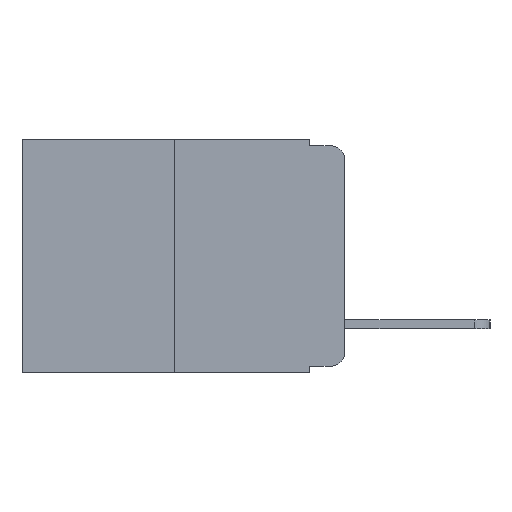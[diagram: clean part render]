
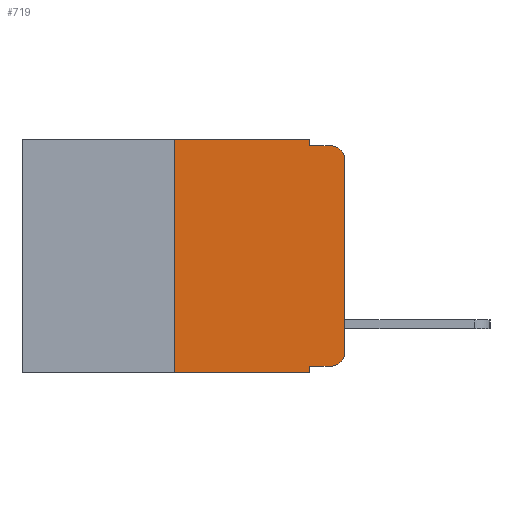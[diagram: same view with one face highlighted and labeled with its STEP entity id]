
A CAD part, left-side view. The second image highlights one B-rep face of the part: STEP entity #719.
In plain terms, the highlighted planar face has unit normal (-1, 0, 0).
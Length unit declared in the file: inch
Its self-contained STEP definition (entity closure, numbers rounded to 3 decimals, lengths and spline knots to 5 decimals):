
#85 = DIRECTION ( 'NONE',  ( 0., 0., 1. ) ) ;
#147 = ORIENTED_EDGE ( 'NONE', *, *, #9426, .F. ) ;
#243 = AXIS2_PLACEMENT_3D ( 'NONE', #4914, #6221, #6185 ) ;
#519 = FACE_OUTER_BOUND ( 'NONE', #11631, .T. ) ;
#551 = EDGE_CURVE ( 'NONE', #7338, #7774, #8680, .T. ) ;
#719 = ADVANCED_FACE ( 'NONE', ( #519 ), #4931, .F. ) ;
#1173 = DIRECTION ( 'NONE',  ( 0., -1., 0. ) ) ;
#1215 = ORIENTED_EDGE ( 'NONE', *, *, #3487, .T. ) ;
#1494 = CARTESIAN_POINT ( 'NONE',  ( 0., 0.02, -0.333 ) ) ;
#1681 = EDGE_CURVE ( 'NONE', #10068, #3542, #5130, .T. ) ;
#1827 = CARTESIAN_POINT ( 'NONE',  ( 0., 0.25, 0. ) ) ;
#1839 = CARTESIAN_POINT ( 'NONE',  ( 0., 0.02, -0.313 ) ) ;
#1917 = VECTOR ( 'NONE', #4175, 39.37008 ) ;
#1948 = CARTESIAN_POINT ( 'NONE',  ( 0., 0.02, -0.03 ) ) ;
#1987 = CIRCLE ( 'NONE', #7078, 0.02 ) ;
#2053 = EDGE_CURVE ( 'NONE', #7774, #11723, #11647, .T. ) ;
#2371 = CARTESIAN_POINT ( 'NONE',  ( 0., 0., 0. ) ) ;
#2797 = VECTOR ( 'NONE', #3889, 39.37008 ) ;
#2840 = CIRCLE ( 'NONE', #4046, 0.02 ) ;
#2930 = DIRECTION ( 'NONE',  ( 0., 0., -1. ) ) ;
#2997 = DIRECTION ( 'NONE',  ( 0., -1., 0. ) ) ;
#3046 = DIRECTION ( 'NONE',  ( 0., 0., -1. ) ) ;
#3122 = ORIENTED_EDGE ( 'NONE', *, *, #8035, .T. ) ;
#3487 = EDGE_CURVE ( 'NONE', #10880, #11723, #2840, .T. ) ;
#3542 = VERTEX_POINT ( 'NONE', #11467 ) ;
#3755 = EDGE_CURVE ( 'NONE', #8293, #7015, #1987, .T. ) ;
#3889 = DIRECTION ( 'NONE',  ( 0., -1., 0. ) ) ;
#3896 = VERTEX_POINT ( 'NONE', #4187 ) ;
#4046 = AXIS2_PLACEMENT_3D ( 'NONE', #1948, #8791, #3046 ) ;
#4175 = DIRECTION ( 'NONE',  ( 0., 0., -1. ) ) ;
#4187 = CARTESIAN_POINT ( 'NONE',  ( 0., 0.25, 0. ) ) ;
#4394 = CARTESIAN_POINT ( 'NONE',  ( 0., 0.473, -0.343 ) ) ;
#4571 = CARTESIAN_POINT ( 'NONE',  ( 0., 0.051, 0. ) ) ;
#4580 = ORIENTED_EDGE ( 'NONE', *, *, #5745, .T. ) ;
#4914 = CARTESIAN_POINT ( 'NONE',  ( 0., 0.473, 0. ) ) ;
#4931 = PLANE ( 'NONE',  #243 ) ;
#5130 = LINE ( 'NONE', #4394, #11792 ) ;
#5489 = LINE ( 'NONE', #8634, #2797 ) ;
#5745 = EDGE_CURVE ( 'NONE', #9624, #8293, #5489, .T. ) ;
#6185 = DIRECTION ( 'NONE',  ( 0., 0., -1. ) ) ;
#6221 = DIRECTION ( 'NONE',  ( 1., 0., 0. ) ) ;
#6591 = DIRECTION ( 'NONE',  ( 0., 0., -1. ) ) ;
#6939 = CARTESIAN_POINT ( 'NONE',  ( 0., 0.473, 0. ) ) ;
#7015 = VERTEX_POINT ( 'NONE', #11472 ) ;
#7027 = EDGE_CURVE ( 'NONE', #9624, #3542, #10163, .T. ) ;
#7057 = CARTESIAN_POINT ( 'NONE',  ( 0., 0.051, -0.01 ) ) ;
#7078 = AXIS2_PLACEMENT_3D ( 'NONE', #1839, #8701, #2930 ) ;
#7101 = VECTOR ( 'NONE', #2997, 39.37008 ) ;
#7279 = ORIENTED_EDGE ( 'NONE', *, *, #551, .F. ) ;
#7338 = VERTEX_POINT ( 'NONE', #4571 ) ;
#7583 = CARTESIAN_POINT ( 'NONE',  ( 0., 0., -0.03 ) ) ;
#7693 = EDGE_CURVE ( 'NONE', #3896, #7338, #11795, .T. ) ;
#7774 = VERTEX_POINT ( 'NONE', #7057 ) ;
#8035 = EDGE_CURVE ( 'NONE', #7015, #10880, #8782, .T. ) ;
#8293 = VERTEX_POINT ( 'NONE', #1494 ) ;
#8555 = ORIENTED_EDGE ( 'NONE', *, *, #1681, .T. ) ;
#8634 = CARTESIAN_POINT ( 'NONE',  ( 0., 0.051, -0.333 ) ) ;
#8680 = LINE ( 'NONE', #10126, #10164 ) ;
#8701 = DIRECTION ( 'NONE',  ( -1., 0., 0. ) ) ;
#8782 = LINE ( 'NONE', #2371, #10535 ) ;
#8791 = DIRECTION ( 'NONE',  ( -1., 0., 0. ) ) ;
#8812 = CARTESIAN_POINT ( 'NONE',  ( 0., 0.02, -0.01 ) ) ;
#8862 = DIRECTION ( 'NONE',  ( 0., -1., 0. ) ) ;
#8869 = CARTESIAN_POINT ( 'NONE',  ( 0., 0.051, 0. ) ) ;
#9307 = VECTOR ( 'NONE', #8862, 39.37008 ) ;
#9351 = ORIENTED_EDGE ( 'NONE', *, *, #2053, .F. ) ;
#9359 = CARTESIAN_POINT ( 'NONE',  ( 0., 0.25, -0.343 ) ) ;
#9426 = EDGE_CURVE ( 'NONE', #10068, #3896, #12198, .T. ) ;
#9624 = VERTEX_POINT ( 'NONE', #9800 ) ;
#9800 = CARTESIAN_POINT ( 'NONE',  ( 0., 0.051, -0.333 ) ) ;
#9886 = VECTOR ( 'NONE', #11361, 39.37008 ) ;
#9903 = ORIENTED_EDGE ( 'NONE', *, *, #7693, .F. ) ;
#10068 = VERTEX_POINT ( 'NONE', #9359 ) ;
#10126 = CARTESIAN_POINT ( 'NONE',  ( 0., 0.051, 0. ) ) ;
#10163 = LINE ( 'NONE', #8869, #1917 ) ;
#10164 = VECTOR ( 'NONE', #6591, 39.37008 ) ;
#10177 = ORIENTED_EDGE ( 'NONE', *, *, #7027, .F. ) ;
#10321 = ORIENTED_EDGE ( 'NONE', *, *, #3755, .T. ) ;
#10535 = VECTOR ( 'NONE', #85, 39.37008 ) ;
#10559 = CARTESIAN_POINT ( 'NONE',  ( 0., 0.051, -0.01 ) ) ;
#10880 = VERTEX_POINT ( 'NONE', #7583 ) ;
#11361 = DIRECTION ( 'NONE',  ( 0., 0., 1. ) ) ;
#11467 = CARTESIAN_POINT ( 'NONE',  ( 0., 0.051, -0.343 ) ) ;
#11472 = CARTESIAN_POINT ( 'NONE',  ( 0., 0., -0.313 ) ) ;
#11631 = EDGE_LOOP ( 'NONE', ( #3122, #1215, #9351, #7279, #9903, #147, #8555, #10177, #4580, #10321 ) ) ;
#11647 = LINE ( 'NONE', #10559, #9307 ) ;
#11723 = VERTEX_POINT ( 'NONE', #8812 ) ;
#11792 = VECTOR ( 'NONE', #1173, 39.37008 ) ;
#11795 = LINE ( 'NONE', #6939, #7101 ) ;
#12198 = LINE ( 'NONE', #1827, #9886 ) ;
